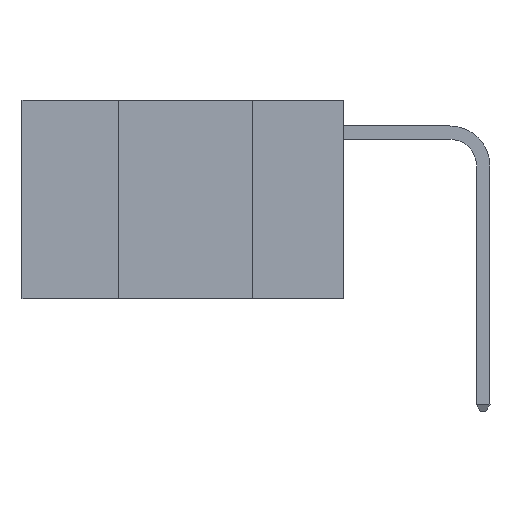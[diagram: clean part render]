
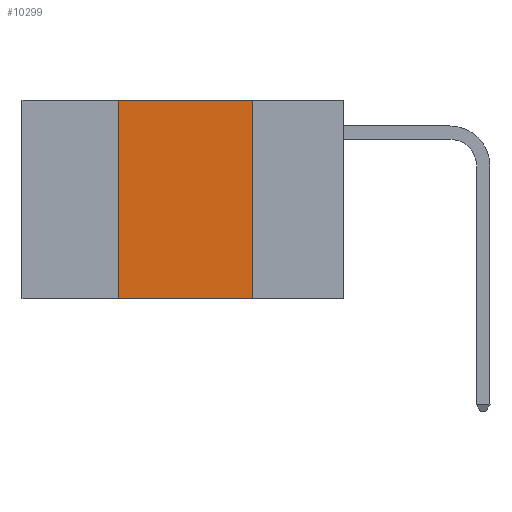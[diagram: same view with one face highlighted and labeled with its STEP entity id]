
A CAD part, left-side view. The second image highlights one B-rep face of the part: STEP entity #10299.
In plain terms, the highlighted planar face has unit normal (-1, 0, 0).
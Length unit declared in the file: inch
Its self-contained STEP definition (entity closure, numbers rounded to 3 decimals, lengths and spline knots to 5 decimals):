
#5 = VERTEX_POINT ( 'NONE', #7522 ) ;
#673 = CARTESIAN_POINT ( 'NONE',  ( 0., 0.6, -0.37 ) ) ;
#852 = LINE ( 'NONE', #673, #9815 ) ;
#855 = VERTEX_POINT ( 'NONE', #7051 ) ;
#964 = VERTEX_POINT ( 'NONE', #1892 ) ;
#1678 = EDGE_LOOP ( 'NONE', ( #8236, #3867, #3448, #8915 ) ) ;
#1762 = LINE ( 'NONE', #3531, #10007 ) ;
#1865 = CARTESIAN_POINT ( 'NONE',  ( 0., 0.6, 0. ) ) ;
#1892 = CARTESIAN_POINT ( 'NONE',  ( 0., 0.42, -0.37 ) ) ;
#1987 = DIRECTION ( 'NONE',  ( 0., 0., 1. ) ) ;
#2070 = AXIS2_PLACEMENT_3D ( 'NONE', #1865, #8311, #3808 ) ;
#2932 = CARTESIAN_POINT ( 'NONE',  ( 0., 0.17, 0. ) ) ;
#3416 = VERTEX_POINT ( 'NONE', #2932 ) ;
#3448 = ORIENTED_EDGE ( 'NONE', *, *, #11224, .F. ) ;
#3459 = CARTESIAN_POINT ( 'NONE',  ( 0., 0.6, 0. ) ) ;
#3531 = CARTESIAN_POINT ( 'NONE',  ( 0., 0.17, 0. ) ) ;
#3760 = VECTOR ( 'NONE', #10674, 39.37008 ) ;
#3808 = DIRECTION ( 'NONE',  ( 0., 0., -1. ) ) ;
#3867 = ORIENTED_EDGE ( 'NONE', *, *, #8867, .F. ) ;
#4298 = DIRECTION ( 'NONE',  ( 0., -1., 0. ) ) ;
#4690 = PLANE ( 'NONE',  #2070 ) ;
#5382 = DIRECTION ( 'NONE',  ( 0., 0., -1. ) ) ;
#5726 = LINE ( 'NONE', #10085, #6419 ) ;
#6338 = FACE_OUTER_BOUND ( 'NONE', #1678, .T. ) ;
#6419 = VECTOR ( 'NONE', #1987, 39.37008 ) ;
#7051 = CARTESIAN_POINT ( 'NONE',  ( 0., 0.17, -0.37 ) ) ;
#7522 = CARTESIAN_POINT ( 'NONE',  ( 0., 0.42, 0. ) ) ;
#7971 = LINE ( 'NONE', #3459, #3760 ) ;
#8236 = ORIENTED_EDGE ( 'NONE', *, *, #11118, .F. ) ;
#8311 = DIRECTION ( 'NONE',  ( 1., 0., 0. ) ) ;
#8867 = EDGE_CURVE ( 'NONE', #5, #3416, #7971, .T. ) ;
#8915 = ORIENTED_EDGE ( 'NONE', *, *, #11519, .T. ) ;
#9815 = VECTOR ( 'NONE', #4298, 39.37008 ) ;
#10007 = VECTOR ( 'NONE', #5382, 39.37008 ) ;
#10085 = CARTESIAN_POINT ( 'NONE',  ( 0., 0.42, 0. ) ) ;
#10299 = ADVANCED_FACE ( 'NONE', ( #6338 ), #4690, .F. ) ;
#10674 = DIRECTION ( 'NONE',  ( 0., -1., 0. ) ) ;
#11118 = EDGE_CURVE ( 'NONE', #3416, #855, #1762, .T. ) ;
#11224 = EDGE_CURVE ( 'NONE', #964, #5, #5726, .T. ) ;
#11519 = EDGE_CURVE ( 'NONE', #964, #855, #852, .T. ) ;
